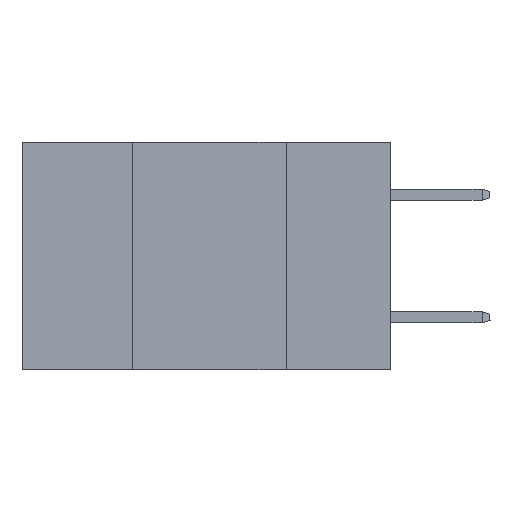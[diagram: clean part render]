
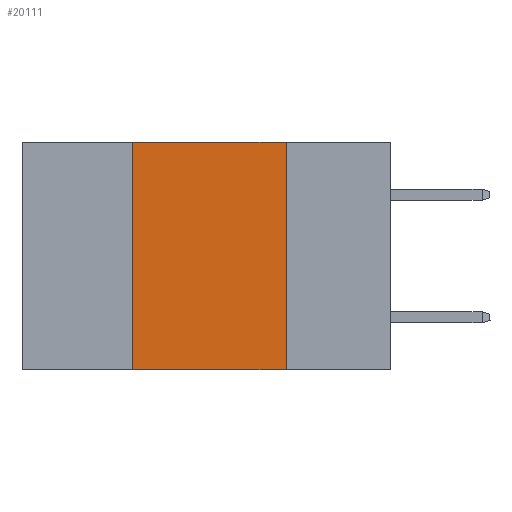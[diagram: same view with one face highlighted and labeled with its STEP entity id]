
A CAD part, left-side view. The second image highlights one B-rep face of the part: STEP entity #20111.
In plain terms, the highlighted planar face has unit normal (-1, 0, 0).
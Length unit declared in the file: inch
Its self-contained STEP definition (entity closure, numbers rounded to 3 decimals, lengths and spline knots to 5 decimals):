
#62 = AXIS2_PLACEMENT_3D ( 'NONE', #43689, #37314, #23155 ) ;
#80 = VECTOR ( 'NONE', #8569, 39.37008 ) ;
#243 = EDGE_CURVE ( 'NONE', #18566, #32670, #3815, .T. ) ;
#318 = CARTESIAN_POINT ( 'NONE',  ( 0., 0.42, 0. ) ) ;
#438 = ORIENTED_EDGE ( 'NONE', *, *, #243, .F. ) ;
#3815 = LINE ( 'NONE', #32641, #5819 ) ;
#4172 = VECTOR ( 'NONE', #20033, 39.37008 ) ;
#5819 = VECTOR ( 'NONE', #25544, 39.37008 ) ;
#5891 = EDGE_CURVE ( 'NONE', #18566, #35005, #27056, .T. ) ;
#6635 = CARTESIAN_POINT ( 'NONE',  ( 0., 0.42, -0.37 ) ) ;
#6841 = CARTESIAN_POINT ( 'NONE',  ( 0., 0.17, -0.37 ) ) ;
#8569 = DIRECTION ( 'NONE',  ( 0., 0., -1. ) ) ;
#9111 = CARTESIAN_POINT ( 'NONE',  ( 0., 0.6, -0.37 ) ) ;
#16707 = VERTEX_POINT ( 'NONE', #44686 ) ;
#16734 = LINE ( 'NONE', #41969, #4172 ) ;
#18320 = ORIENTED_EDGE ( 'NONE', *, *, #35325, .F. ) ;
#18467 = FACE_OUTER_BOUND ( 'NONE', #43030, .T. ) ;
#18566 = VERTEX_POINT ( 'NONE', #6635 ) ;
#20033 = DIRECTION ( 'NONE',  ( 0., -1., 0. ) ) ;
#20111 = ADVANCED_FACE ( 'NONE', ( #18467 ), #32873, .F. ) ;
#23155 = DIRECTION ( 'NONE',  ( 0., 0., -1. ) ) ;
#23504 = DIRECTION ( 'NONE',  ( 0., -1., 0. ) ) ;
#25544 = DIRECTION ( 'NONE',  ( 0., 0., 1. ) ) ;
#27056 = LINE ( 'NONE', #9111, #44345 ) ;
#32641 = CARTESIAN_POINT ( 'NONE',  ( 0., 0.42, 0. ) ) ;
#32670 = VERTEX_POINT ( 'NONE', #318 ) ;
#32873 = PLANE ( 'NONE',  #62 ) ;
#35005 = VERTEX_POINT ( 'NONE', #6841 ) ;
#35325 = EDGE_CURVE ( 'NONE', #32670, #16707, #16734, .T. ) ;
#37314 = DIRECTION ( 'NONE',  ( 1., 0., 0. ) ) ;
#40656 = CARTESIAN_POINT ( 'NONE',  ( 0., 0.17, 0. ) ) ;
#41347 = LINE ( 'NONE', #40656, #80 ) ;
#41969 = CARTESIAN_POINT ( 'NONE',  ( 0., 0.6, 0. ) ) ;
#43030 = EDGE_LOOP ( 'NONE', ( #43806, #18320, #438, #46466 ) ) ;
#43689 = CARTESIAN_POINT ( 'NONE',  ( 0., 0.6, 0. ) ) ;
#43806 = ORIENTED_EDGE ( 'NONE', *, *, #45491, .F. ) ;
#44345 = VECTOR ( 'NONE', #23504, 39.37008 ) ;
#44686 = CARTESIAN_POINT ( 'NONE',  ( 0., 0.17, 0. ) ) ;
#45491 = EDGE_CURVE ( 'NONE', #16707, #35005, #41347, .T. ) ;
#46466 = ORIENTED_EDGE ( 'NONE', *, *, #5891, .T. ) ;
